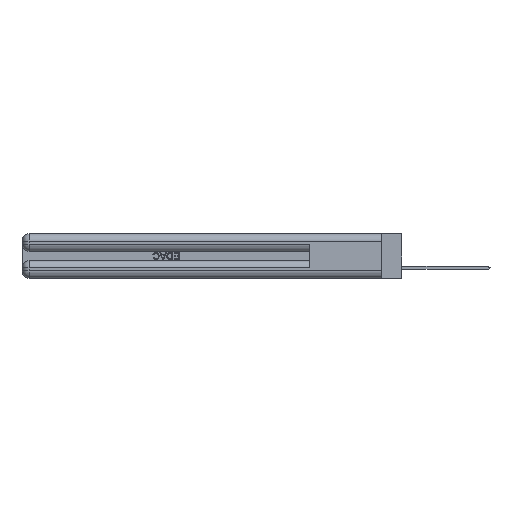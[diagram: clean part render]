
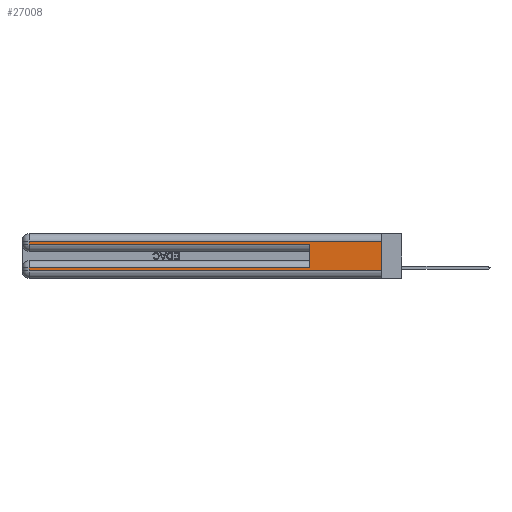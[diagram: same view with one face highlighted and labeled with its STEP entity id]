
A CAD part, left-side view. The second image highlights one B-rep face of the part: STEP entity #27008.
In plain terms, the highlighted planar face has unit normal (-1, 0, 0).
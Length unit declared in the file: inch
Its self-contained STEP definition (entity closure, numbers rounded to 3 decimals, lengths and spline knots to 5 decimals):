
#193 = VERTEX_POINT ( 'NONE', #24810 ) ;
#2429 = CARTESIAN_POINT ( 'NONE',  ( 0., 0., 0.37 ) ) ;
#2488 = VECTOR ( 'NONE', #12114, 39.37008 ) ;
#3033 = CARTESIAN_POINT ( 'NONE',  ( 0., 2.94, 0.085 ) ) ;
#3500 = CARTESIAN_POINT ( 'NONE',  ( 0., 0., 0.285 ) ) ;
#3631 = DIRECTION ( 'NONE',  ( 0., -1., 0. ) ) ;
#4198 = LINE ( 'NONE', #37722, #37037 ) ;
#4399 = VERTEX_POINT ( 'NONE', #20960 ) ;
#5840 = DIRECTION ( 'NONE',  ( 1., 0., 0. ) ) ;
#6168 = LINE ( 'NONE', #19397, #13491 ) ;
#7571 = FACE_OUTER_BOUND ( 'NONE', #19019, .T. ) ;
#7845 = LINE ( 'NONE', #34404, #23795 ) ;
#8294 = CARTESIAN_POINT ( 'NONE',  ( 0., 0., 0.06 ) ) ;
#8915 = ORIENTED_EDGE ( 'NONE', *, *, #30211, .T. ) ;
#8924 = DIRECTION ( 'NONE',  ( 0., 1., 0. ) ) ;
#9493 = CARTESIAN_POINT ( 'NONE',  ( 0., 0., 0.06 ) ) ;
#9526 = CARTESIAN_POINT ( 'NONE',  ( 0., 2.94, 0.37 ) ) ;
#10729 = LINE ( 'NONE', #9526, #12998 ) ;
#12114 = DIRECTION ( 'NONE',  ( 0., 1., 0. ) ) ;
#12232 = ORIENTED_EDGE ( 'NONE', *, *, #15512, .T. ) ;
#12998 = VECTOR ( 'NONE', #13299, 39.37008 ) ;
#13299 = DIRECTION ( 'NONE',  ( 0., 0., -1. ) ) ;
#13491 = VECTOR ( 'NONE', #26241, 39.37008 ) ;
#13649 = ORIENTED_EDGE ( 'NONE', *, *, #29391, .T. ) ;
#14694 = ORIENTED_EDGE ( 'NONE', *, *, #18992, .F. ) ;
#15512 = EDGE_CURVE ( 'NONE', #18880, #17323, #34016, .T. ) ;
#15866 = LINE ( 'NONE', #3500, #31290 ) ;
#16218 = ORIENTED_EDGE ( 'NONE', *, *, #16842, .F. ) ;
#16298 = DIRECTION ( 'NONE',  ( 0., 0., -1. ) ) ;
#16719 = PLANE ( 'NONE',  #45133 ) ;
#16842 = EDGE_CURVE ( 'NONE', #28447, #17323, #6168, .T. ) ;
#17323 = VERTEX_POINT ( 'NONE', #9493 ) ;
#17483 = VERTEX_POINT ( 'NONE', #3033 ) ;
#18231 = VERTEX_POINT ( 'NONE', #26474 ) ;
#18553 = ORIENTED_EDGE ( 'NONE', *, *, #34210, .T. ) ;
#18647 = VERTEX_POINT ( 'NONE', #20844 ) ;
#18880 = VERTEX_POINT ( 'NONE', #43667 ) ;
#18992 = EDGE_CURVE ( 'NONE', #18231, #18647, #44992, .T. ) ;
#19019 = EDGE_LOOP ( 'NONE', ( #16218, #39548, #13649, #18553, #14694, #41387, #8915, #12232 ) ) ;
#19397 = CARTESIAN_POINT ( 'NONE',  ( 0., 0., 0.37 ) ) ;
#20844 = CARTESIAN_POINT ( 'NONE',  ( 0., 0.6, 0.285 ) ) ;
#20960 = CARTESIAN_POINT ( 'NONE',  ( 0., 2.94, 0.285 ) ) ;
#23243 = CARTESIAN_POINT ( 'NONE',  ( 0., 0., 0.31 ) ) ;
#23795 = VECTOR ( 'NONE', #16298, 39.37008 ) ;
#24810 = CARTESIAN_POINT ( 'NONE',  ( 0., 2.94, 0.31 ) ) ;
#26241 = DIRECTION ( 'NONE',  ( 0., 0., -1. ) ) ;
#26474 = CARTESIAN_POINT ( 'NONE',  ( 0., 0.6, 0.085 ) ) ;
#27008 = ADVANCED_FACE ( 'NONE', ( #7571 ), #16719, .F. ) ;
#27220 = EDGE_CURVE ( 'NONE', #18231, #17483, #4198, .T. ) ;
#27717 = DIRECTION ( 'NONE',  ( 0., 0., -1. ) ) ;
#28447 = VERTEX_POINT ( 'NONE', #23243 ) ;
#29391 = EDGE_CURVE ( 'NONE', #193, #4399, #10729, .T. ) ;
#30211 = EDGE_CURVE ( 'NONE', #17483, #18880, #7845, .T. ) ;
#31290 = VECTOR ( 'NONE', #3631, 39.37008 ) ;
#33318 = CARTESIAN_POINT ( 'NONE',  ( 0., 0.6, 0.145 ) ) ;
#33673 = VECTOR ( 'NONE', #33797, 39.37008 ) ;
#33791 = CARTESIAN_POINT ( 'NONE',  ( 0., 0., 0.31 ) ) ;
#33796 = EDGE_CURVE ( 'NONE', #28447, #193, #46592, .T. ) ;
#33797 = DIRECTION ( 'NONE',  ( 0., 0., 1. ) ) ;
#34016 = LINE ( 'NONE', #8294, #45364 ) ;
#34210 = EDGE_CURVE ( 'NONE', #4399, #18647, #15866, .T. ) ;
#34404 = CARTESIAN_POINT ( 'NONE',  ( 0., 2.94, 0.37 ) ) ;
#37037 = VECTOR ( 'NONE', #8924, 39.37008 ) ;
#37722 = CARTESIAN_POINT ( 'NONE',  ( 0., 0., 0.085 ) ) ;
#39548 = ORIENTED_EDGE ( 'NONE', *, *, #33796, .T. ) ;
#40282 = DIRECTION ( 'NONE',  ( 0., -1., 0. ) ) ;
#41387 = ORIENTED_EDGE ( 'NONE', *, *, #27220, .T. ) ;
#43667 = CARTESIAN_POINT ( 'NONE',  ( 0., 2.94, 0.06 ) ) ;
#44992 = LINE ( 'NONE', #33318, #33673 ) ;
#45133 = AXIS2_PLACEMENT_3D ( 'NONE', #2429, #5840, #27717 ) ;
#45364 = VECTOR ( 'NONE', #40282, 39.37008 ) ;
#46592 = LINE ( 'NONE', #33791, #2488 ) ;
